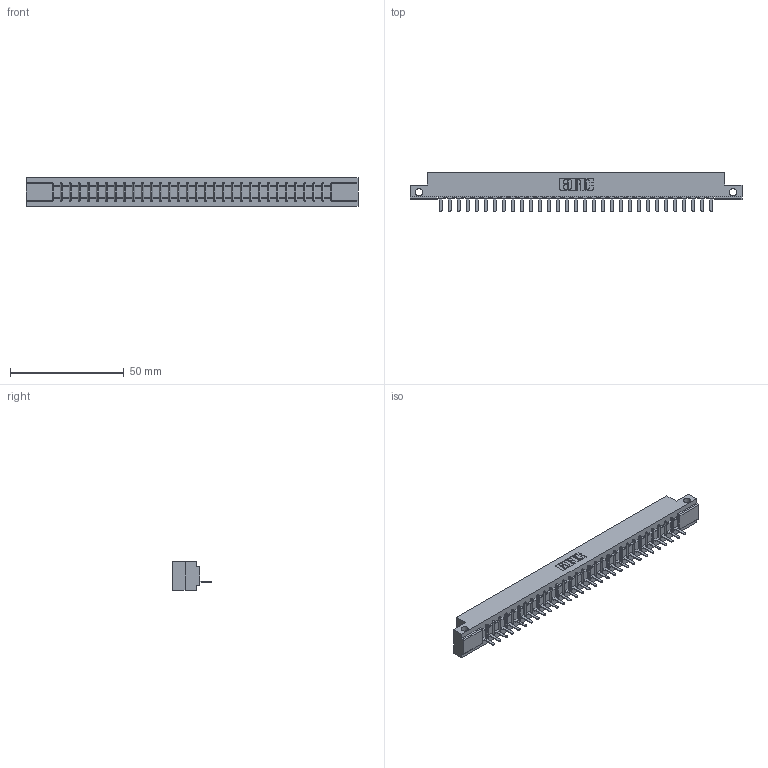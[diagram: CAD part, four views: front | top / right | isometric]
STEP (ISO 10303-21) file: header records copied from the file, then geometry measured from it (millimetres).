
FILE_DESCRIPTION (( 'STEP AP203' ), '1' );
FILE_NAME ('357-031-421-112.STEP', '2020-10-02T03:40:03', ( '' ), ( '' ), 'SwSTEP 2.0', 'SolidWorks 2020', '' );
FILE_SCHEMA (( 'CONFIG_CONTROL_DESIGN' ));
Length unit declared in the file: inch
Products named in the file (3): 357-031-421-112; 307 Part_.128 Dia Side Mounting Holes; 307-290-002_521
Assembly tree (32 placements, depth 2):
  357-031-421-112
    307 Part_.128 Dia Side Mounting Holes
    307-290-002_521  x31
Bounding box: 145.85 x 17.42 x 12.7 mm (x, y, z)
Volume: 15385.1 mm3; surface area: 19098.1 mm2
Topology: 32 solids, 32 shells, 2444 faces, 7515 edges, 4922 vertices
Faces by surface type: plane 1465, cylinder 915, sphere 64
Entity records: 28652 total; most frequent: CARTESIAN_POINT 4832, ORIENTED_EDGE 4822, DIRECTION 4699, EDGE_CURVE 2411, LINE 1841, VECTOR 1841, VERTEX_POINT 1562, AXIS2_PLACEMENT_3D 1429
